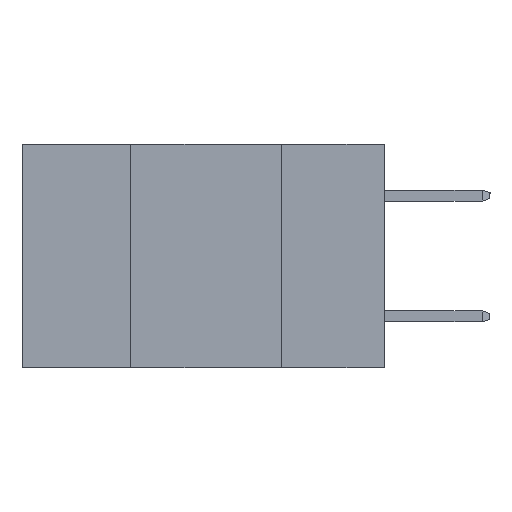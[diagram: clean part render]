
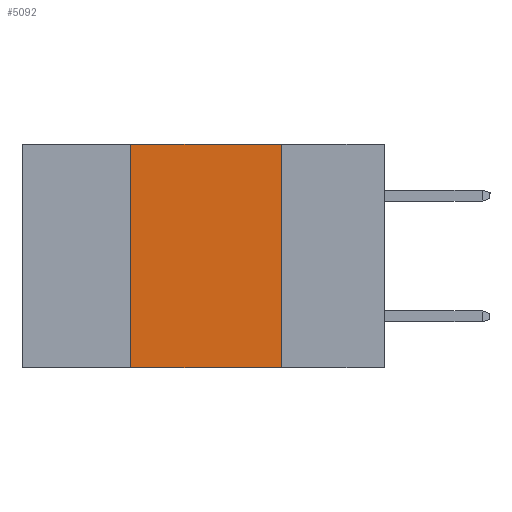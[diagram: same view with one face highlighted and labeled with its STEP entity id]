
A CAD part, left-side view. The second image highlights one B-rep face of the part: STEP entity #5092.
In plain terms, the highlighted planar face has unit normal (-1, 0, 0).
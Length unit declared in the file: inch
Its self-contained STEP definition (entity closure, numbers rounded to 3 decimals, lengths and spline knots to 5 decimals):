
#54 = CARTESIAN_POINT ( 'NONE',  ( 0., 0.6, 0. ) ) ;
#548 = CARTESIAN_POINT ( 'NONE',  ( 0., 0.6, 0. ) ) ;
#629 = DIRECTION ( 'NONE',  ( 0., 0., 1. ) ) ;
#1021 = ORIENTED_EDGE ( 'NONE', *, *, #4537, .T. ) ;
#1716 = VERTEX_POINT ( 'NONE', #5485 ) ;
#2252 = CARTESIAN_POINT ( 'NONE',  ( 0., 0.42, -0.37 ) ) ;
#2276 = DIRECTION ( 'NONE',  ( 0., 0., -1. ) ) ;
#2404 = CARTESIAN_POINT ( 'NONE',  ( 0., 0.42, 0. ) ) ;
#2482 = EDGE_LOOP ( 'NONE', ( #4183, #5389, #7648, #1021 ) ) ;
#3915 = EDGE_CURVE ( 'NONE', #9612, #1716, #5398, .T. ) ;
#4183 = ORIENTED_EDGE ( 'NONE', *, *, #9763, .F. ) ;
#4289 = VECTOR ( 'NONE', #10512, 39.37008 ) ;
#4389 = CARTESIAN_POINT ( 'NONE',  ( 0., 0.42, -0.37 ) ) ;
#4537 = EDGE_CURVE ( 'NONE', #9370, #5661, #11193, .T. ) ;
#5034 = CARTESIAN_POINT ( 'NONE',  ( 0., 0.6, -0.37 ) ) ;
#5092 = ADVANCED_FACE ( 'NONE', ( #6628 ), #10261, .F. ) ;
#5152 = VECTOR ( 'NONE', #629, 39.37008 ) ;
#5389 = ORIENTED_EDGE ( 'NONE', *, *, #3915, .F. ) ;
#5398 = LINE ( 'NONE', #54, #7128 ) ;
#5485 = CARTESIAN_POINT ( 'NONE',  ( 0., 0.17, 0. ) ) ;
#5637 = LINE ( 'NONE', #2252, #5152 ) ;
#5661 = VERTEX_POINT ( 'NONE', #9388 ) ;
#6307 = DIRECTION ( 'NONE',  ( 0., -1., 0. ) ) ;
#6401 = VECTOR ( 'NONE', #8490, 39.37008 ) ;
#6591 = AXIS2_PLACEMENT_3D ( 'NONE', #548, #8476, #2276 ) ;
#6628 = FACE_OUTER_BOUND ( 'NONE', #2482, .T. ) ;
#6989 = LINE ( 'NONE', #7835, #4289 ) ;
#7128 = VECTOR ( 'NONE', #6307, 39.37008 ) ;
#7415 = EDGE_CURVE ( 'NONE', #9370, #9612, #5637, .T. ) ;
#7648 = ORIENTED_EDGE ( 'NONE', *, *, #7415, .F. ) ;
#7835 = CARTESIAN_POINT ( 'NONE',  ( 0., 0.17, -0.37 ) ) ;
#8476 = DIRECTION ( 'NONE',  ( 1., 0., 0. ) ) ;
#8490 = DIRECTION ( 'NONE',  ( 0., -1., 0. ) ) ;
#9370 = VERTEX_POINT ( 'NONE', #4389 ) ;
#9388 = CARTESIAN_POINT ( 'NONE',  ( 0., 0.17, -0.37 ) ) ;
#9612 = VERTEX_POINT ( 'NONE', #2404 ) ;
#9763 = EDGE_CURVE ( 'NONE', #1716, #5661, #6989, .T. ) ;
#10261 = PLANE ( 'NONE',  #6591 ) ;
#10512 = DIRECTION ( 'NONE',  ( 0., 0., -1. ) ) ;
#11193 = LINE ( 'NONE', #5034, #6401 ) ;
